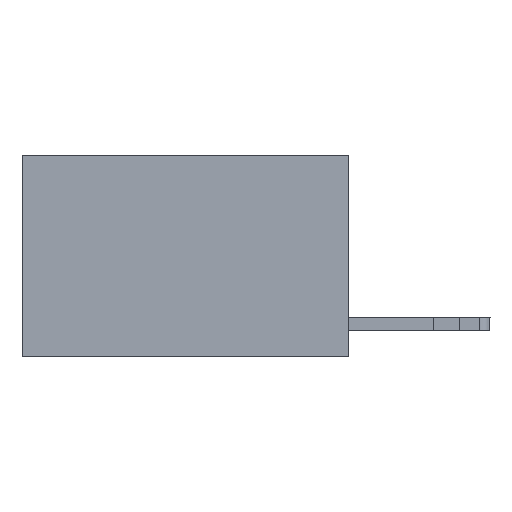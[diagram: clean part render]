
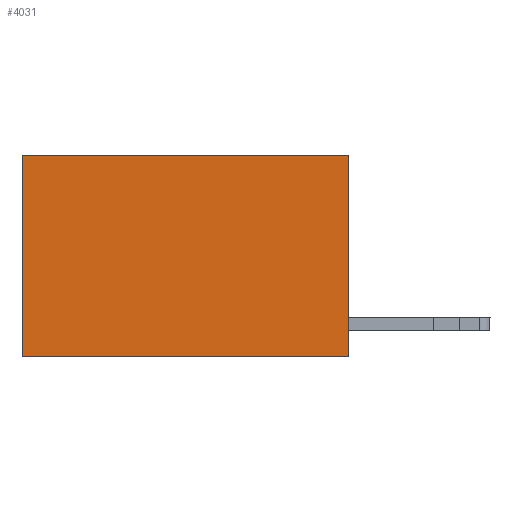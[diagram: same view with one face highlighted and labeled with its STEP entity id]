
A CAD part, left-side view. The second image highlights one B-rep face of the part: STEP entity #4031.
In plain terms, the highlighted planar face has unit normal (-1, 0, 0).
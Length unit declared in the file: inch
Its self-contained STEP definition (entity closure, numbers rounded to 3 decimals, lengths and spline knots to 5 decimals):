
#898 = ORIENTED_EDGE ( 'NONE', *, *, #8984, .T. ) ;
#2588 = AXIS2_PLACEMENT_3D ( 'NONE', #19601, #13774, #4468 ) ;
#2845 = PLANE ( 'NONE',  #2588 ) ;
#3356 = VERTEX_POINT ( 'NONE', #18990 ) ;
#3473 = EDGE_CURVE ( 'NONE', #3356, #3718, #18914, .T. ) ;
#3474 = EDGE_CURVE ( 'NONE', #3951, #3718, #19365, .T. ) ;
#3493 = EDGE_LOOP ( 'NONE', ( #13579, #3755, #15777, #898 ) ) ;
#3718 = VERTEX_POINT ( 'NONE', #19152 ) ;
#3755 = ORIENTED_EDGE ( 'NONE', *, *, #3474, .F. ) ;
#3951 = VERTEX_POINT ( 'NONE', #13578 ) ;
#4031 = ADVANCED_FACE ( 'NONE', ( #15004 ), #2845, .F. ) ;
#4109 = VERTEX_POINT ( 'NONE', #18298 ) ;
#4468 = DIRECTION ( 'NONE',  ( 0., 0., -1. ) ) ;
#4976 = LINE ( 'NONE', #13911, #9185 ) ;
#6375 = LINE ( 'NONE', #11899, #10044 ) ;
#6935 = VECTOR ( 'NONE', #11108, 39.37008 ) ;
#7828 = DIRECTION ( 'NONE',  ( 0., 1., 0. ) ) ;
#8984 = EDGE_CURVE ( 'NONE', #4109, #3356, #4976, .T. ) ;
#9185 = VECTOR ( 'NONE', #7828, 39.37008 ) ;
#10044 = VECTOR ( 'NONE', #14895, 39.37008 ) ;
#11108 = DIRECTION ( 'NONE',  ( 0., 0., -1. ) ) ;
#11899 = CARTESIAN_POINT ( 'NONE',  ( 0.2625, 0., 0. ) ) ;
#12791 = CARTESIAN_POINT ( 'NONE',  ( 0.2625, 0., -0.37 ) ) ;
#13578 = CARTESIAN_POINT ( 'NONE',  ( 0.2625, 0., -0.37 ) ) ;
#13579 = ORIENTED_EDGE ( 'NONE', *, *, #3473, .T. ) ;
#13611 = DIRECTION ( 'NONE',  ( 0., 1., 0. ) ) ;
#13774 = DIRECTION ( 'NONE',  ( 1., 0., 0. ) ) ;
#13784 = EDGE_CURVE ( 'NONE', #4109, #3951, #6375, .T. ) ;
#13911 = CARTESIAN_POINT ( 'NONE',  ( 0.2625, 0., 0. ) ) ;
#14895 = DIRECTION ( 'NONE',  ( 0., 0., -1. ) ) ;
#15004 = FACE_OUTER_BOUND ( 'NONE', #3493, .T. ) ;
#15777 = ORIENTED_EDGE ( 'NONE', *, *, #13784, .F. ) ;
#17932 = CARTESIAN_POINT ( 'NONE',  ( 0.2625, 0.6, 0. ) ) ;
#18298 = CARTESIAN_POINT ( 'NONE',  ( 0.2625, 0., 0. ) ) ;
#18441 = VECTOR ( 'NONE', #13611, 39.37008 ) ;
#18914 = LINE ( 'NONE', #17932, #6935 ) ;
#18990 = CARTESIAN_POINT ( 'NONE',  ( 0.2625, 0.6, 0. ) ) ;
#19152 = CARTESIAN_POINT ( 'NONE',  ( 0.2625, 0.6, -0.37 ) ) ;
#19365 = LINE ( 'NONE', #12791, #18441 ) ;
#19601 = CARTESIAN_POINT ( 'NONE',  ( 0.2625, 0., 0. ) ) ;
